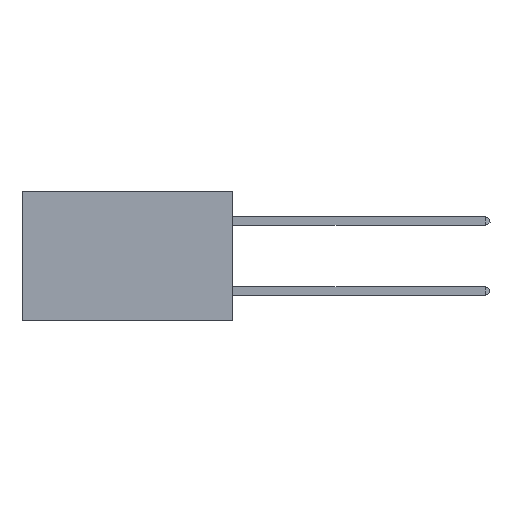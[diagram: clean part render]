
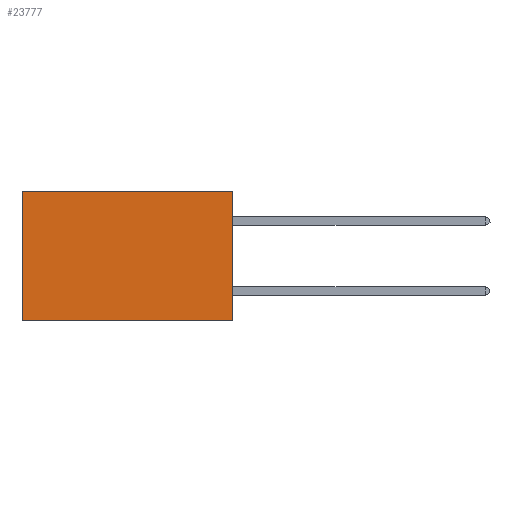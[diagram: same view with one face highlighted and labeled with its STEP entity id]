
A CAD part, left-side view. The second image highlights one B-rep face of the part: STEP entity #23777.
In plain terms, the highlighted planar face has unit normal (-1, 0, 0).
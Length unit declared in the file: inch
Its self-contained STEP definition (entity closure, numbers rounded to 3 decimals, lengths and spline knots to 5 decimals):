
#4899 = VERTEX_POINT ( 'NONE', #8409 ) ;
#5020 = CARTESIAN_POINT ( 'NONE',  ( 0.2875, 0., 0. ) ) ;
#6275 = LINE ( 'NONE', #12930, #15324 ) ;
#7568 = DIRECTION ( 'NONE',  ( 0., 0., -1. ) ) ;
#7721 = VECTOR ( 'NONE', #26048, 39.37008 ) ;
#8409 = CARTESIAN_POINT ( 'NONE',  ( 0.2875, 0.6, -0.37 ) ) ;
#9128 = ORIENTED_EDGE ( 'NONE', *, *, #28526, .F. ) ;
#9721 = ORIENTED_EDGE ( 'NONE', *, *, #23857, .T. ) ;
#10017 = CARTESIAN_POINT ( 'NONE',  ( 0.2875, 0., 0. ) ) ;
#10351 = CARTESIAN_POINT ( 'NONE',  ( 0.2875, 0., 0. ) ) ;
#10666 = FACE_OUTER_BOUND ( 'NONE', #27401, .T. ) ;
#10781 = VERTEX_POINT ( 'NONE', #13864 ) ;
#10848 = VECTOR ( 'NONE', #13959, 39.37008 ) ;
#11063 = CARTESIAN_POINT ( 'NONE',  ( 0.2875, 0.6, 0. ) ) ;
#12930 = CARTESIAN_POINT ( 'NONE',  ( 0.2875, 0., 0. ) ) ;
#13864 = CARTESIAN_POINT ( 'NONE',  ( 0.2875, 0.6, 0. ) ) ;
#13959 = DIRECTION ( 'NONE',  ( 0., 1., 0. ) ) ;
#14958 = EDGE_CURVE ( 'NONE', #10781, #4899, #18565, .T. ) ;
#15320 = VERTEX_POINT ( 'NONE', #10351 ) ;
#15324 = VECTOR ( 'NONE', #22263, 39.37008 ) ;
#15410 = EDGE_CURVE ( 'NONE', #15320, #16223, #6275, .T. ) ;
#16223 = VERTEX_POINT ( 'NONE', #21790 ) ;
#16952 = LINE ( 'NONE', #25646, #10848 ) ;
#18160 = ORIENTED_EDGE ( 'NONE', *, *, #15410, .F. ) ;
#18565 = LINE ( 'NONE', #11063, #20733 ) ;
#18693 = ORIENTED_EDGE ( 'NONE', *, *, #14958, .T. ) ;
#20733 = VECTOR ( 'NONE', #22239, 39.37008 ) ;
#21513 = DIRECTION ( 'NONE',  ( 1., 0., 0. ) ) ;
#21790 = CARTESIAN_POINT ( 'NONE',  ( 0.2875, 0., -0.37 ) ) ;
#22239 = DIRECTION ( 'NONE',  ( 0., 0., -1. ) ) ;
#22263 = DIRECTION ( 'NONE',  ( 0., 0., -1. ) ) ;
#23261 = LINE ( 'NONE', #5020, #7721 ) ;
#23777 = ADVANCED_FACE ( 'NONE', ( #10666 ), #28067, .F. ) ;
#23857 = EDGE_CURVE ( 'NONE', #15320, #10781, #23261, .T. ) ;
#25646 = CARTESIAN_POINT ( 'NONE',  ( 0.2875, 0., -0.37 ) ) ;
#26048 = DIRECTION ( 'NONE',  ( 0., 1., 0. ) ) ;
#26658 = AXIS2_PLACEMENT_3D ( 'NONE', #10017, #21513, #7568 ) ;
#27401 = EDGE_LOOP ( 'NONE', ( #18693, #9128, #18160, #9721 ) ) ;
#28067 = PLANE ( 'NONE',  #26658 ) ;
#28526 = EDGE_CURVE ( 'NONE', #16223, #4899, #16952, .T. ) ;
